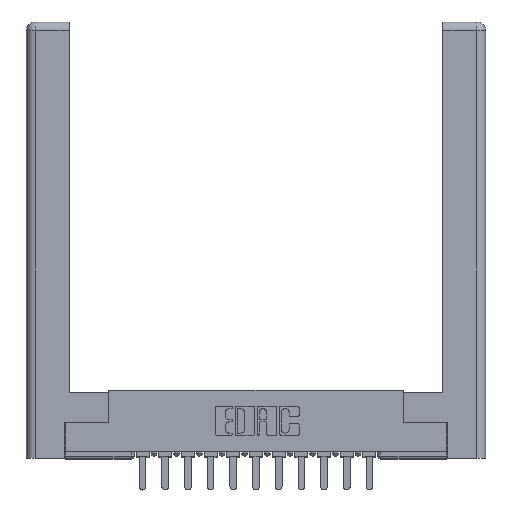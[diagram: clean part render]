
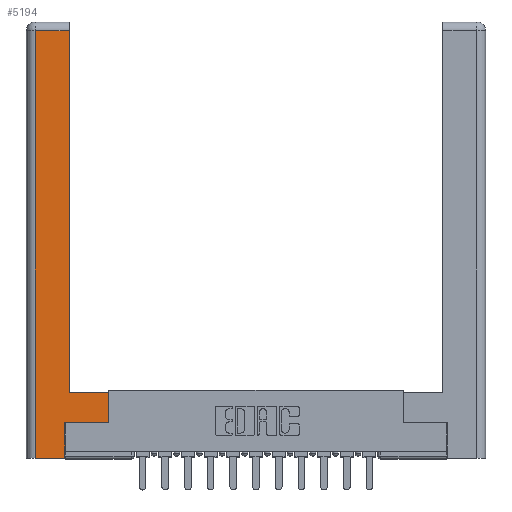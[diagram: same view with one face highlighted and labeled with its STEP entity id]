
A CAD part, top view. The second image highlights one B-rep face of the part: STEP entity #5194.
In plain terms, the highlighted planar face has unit normal (0, 0, 1).
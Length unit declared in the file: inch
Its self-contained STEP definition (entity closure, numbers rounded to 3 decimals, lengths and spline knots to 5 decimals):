
#2 = EDGE_CURVE ( 'NONE', #12241, #13143, #581, .T. ) ;
#255 = DIRECTION ( 'NONE',  ( 1., 0., 0. ) ) ;
#286 = CARTESIAN_POINT ( 'NONE',  ( 0.295, 2.94, 0. ) ) ;
#323 = CARTESIAN_POINT ( 'NONE',  ( 0.0615, 0., 0. ) ) ;
#581 = LINE ( 'NONE', #16080, #15435 ) ;
#951 = DIRECTION ( 'NONE',  ( -1., 0., 0. ) ) ;
#1217 = ORIENTED_EDGE ( 'NONE', *, *, #12962, .T. ) ;
#1642 = CARTESIAN_POINT ( 'NONE',  ( 0.0615, 2.94, 0. ) ) ;
#1805 = VERTEX_POINT ( 'NONE', #12109 ) ;
#1903 = CARTESIAN_POINT ( 'NONE',  ( 0.295, 3., 0. ) ) ;
#2542 = VERTEX_POINT ( 'NONE', #7339 ) ;
#2581 = ORIENTED_EDGE ( 'NONE', *, *, #2, .T. ) ;
#2980 = CARTESIAN_POINT ( 'NONE',  ( 0.565, 0.45, 0. ) ) ;
#3090 = AXIS2_PLACEMENT_3D ( 'NONE', #16112, #4563, #12279 ) ;
#3247 = LINE ( 'NONE', #1903, #15280 ) ;
#3327 = LINE ( 'NONE', #1642, #16558 ) ;
#3794 = ORIENTED_EDGE ( 'NONE', *, *, #13724, .T. ) ;
#4025 = VERTEX_POINT ( 'NONE', #15622 ) ;
#4113 = DIRECTION ( 'NONE',  ( 0., 1., 0. ) ) ;
#4145 = ORIENTED_EDGE ( 'NONE', *, *, #9837, .T. ) ;
#4498 = DIRECTION ( 'NONE',  ( 0., 1., 0. ) ) ;
#4563 = DIRECTION ( 'NONE',  ( 0., 0., -1. ) ) ;
#4685 = EDGE_CURVE ( 'NONE', #9495, #4025, #3327, .T. ) ;
#5067 = VECTOR ( 'NONE', #4113, 39.37008 ) ;
#5194 = ADVANCED_FACE ( 'NONE', ( #12122 ), #5838, .F. ) ;
#5283 = DIRECTION ( 'NONE',  ( 0., 1., 0. ) ) ;
#5550 = LINE ( 'NONE', #12381, #12752 ) ;
#5838 = PLANE ( 'NONE',  #3090 ) ;
#6434 = VECTOR ( 'NONE', #12691, 39.37008 ) ;
#6773 = LINE ( 'NONE', #12967, #12998 ) ;
#7298 = ORIENTED_EDGE ( 'NONE', *, *, #16353, .T. ) ;
#7339 = CARTESIAN_POINT ( 'NONE',  ( 0.265, 0., 0. ) ) ;
#7371 = EDGE_CURVE ( 'NONE', #1805, #12241, #8441, .T. ) ;
#8441 = LINE ( 'NONE', #2980, #5067 ) ;
#8784 = CARTESIAN_POINT ( 'NONE',  ( 0.265, 0.245, 0. ) ) ;
#8850 = DIRECTION ( 'NONE',  ( -1., 0., 0. ) ) ;
#8902 = EDGE_CURVE ( 'NONE', #14500, #1805, #6773, .T. ) ;
#9120 = CARTESIAN_POINT ( 'NONE',  ( 0.295, 0.45, 0. ) ) ;
#9439 = LINE ( 'NONE', #10232, #6434 ) ;
#9495 = VERTEX_POINT ( 'NONE', #286 ) ;
#9837 = EDGE_CURVE ( 'NONE', #4025, #14703, #5550, .T. ) ;
#10232 = CARTESIAN_POINT ( 'NONE',  ( 0.265, 0., 0. ) ) ;
#10299 = CARTESIAN_POINT ( 'NONE',  ( 0.265, 0.245, 0. ) ) ;
#11958 = LINE ( 'NONE', #10299, #15989 ) ;
#12109 = CARTESIAN_POINT ( 'NONE',  ( 0.565, 0.245, 0. ) ) ;
#12122 = FACE_OUTER_BOUND ( 'NONE', #14864, .T. ) ;
#12131 = CARTESIAN_POINT ( 'NONE',  ( 0.565, 0.45, 0. ) ) ;
#12241 = VERTEX_POINT ( 'NONE', #12131 ) ;
#12279 = DIRECTION ( 'NONE',  ( -1., 0., 0. ) ) ;
#12381 = CARTESIAN_POINT ( 'NONE',  ( 0.0615, 0., 0. ) ) ;
#12433 = DIRECTION ( 'NONE',  ( 0., -1., 0. ) ) ;
#12691 = DIRECTION ( 'NONE',  ( 1., 0., 0. ) ) ;
#12740 = ORIENTED_EDGE ( 'NONE', *, *, #8902, .T. ) ;
#12752 = VECTOR ( 'NONE', #12433, 39.37008 ) ;
#12962 = EDGE_CURVE ( 'NONE', #13143, #9495, #3247, .T. ) ;
#12967 = CARTESIAN_POINT ( 'NONE',  ( 0.565, 0.245, 0. ) ) ;
#12998 = VECTOR ( 'NONE', #255, 39.37008 ) ;
#13143 = VERTEX_POINT ( 'NONE', #9120 ) ;
#13724 = EDGE_CURVE ( 'NONE', #14703, #2542, #9439, .T. ) ;
#13774 = ORIENTED_EDGE ( 'NONE', *, *, #4685, .T. ) ;
#14311 = ORIENTED_EDGE ( 'NONE', *, *, #7371, .T. ) ;
#14500 = VERTEX_POINT ( 'NONE', #8784 ) ;
#14703 = VERTEX_POINT ( 'NONE', #323 ) ;
#14864 = EDGE_LOOP ( 'NONE', ( #1217, #13774, #4145, #3794, #7298, #12740, #14311, #2581 ) ) ;
#15280 = VECTOR ( 'NONE', #4498, 39.37008 ) ;
#15435 = VECTOR ( 'NONE', #951, 39.37008 ) ;
#15622 = CARTESIAN_POINT ( 'NONE',  ( 0.0615, 2.94, 0. ) ) ;
#15989 = VECTOR ( 'NONE', #5283, 39.37008 ) ;
#16080 = CARTESIAN_POINT ( 'NONE',  ( 0.295, 0.45, 0. ) ) ;
#16112 = CARTESIAN_POINT ( 'NONE',  ( 0., 0., 0. ) ) ;
#16353 = EDGE_CURVE ( 'NONE', #2542, #14500, #11958, .T. ) ;
#16558 = VECTOR ( 'NONE', #8850, 39.37008 ) ;
